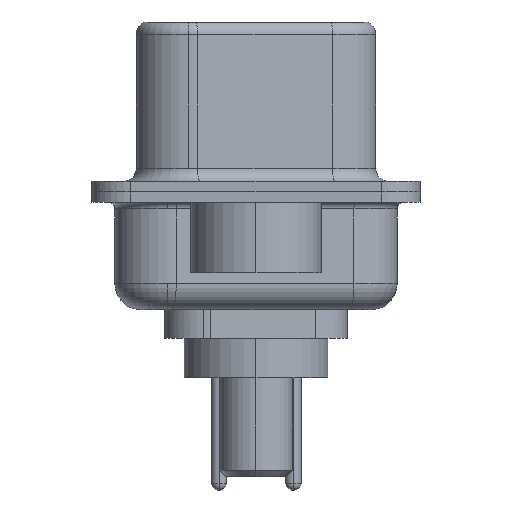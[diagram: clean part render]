
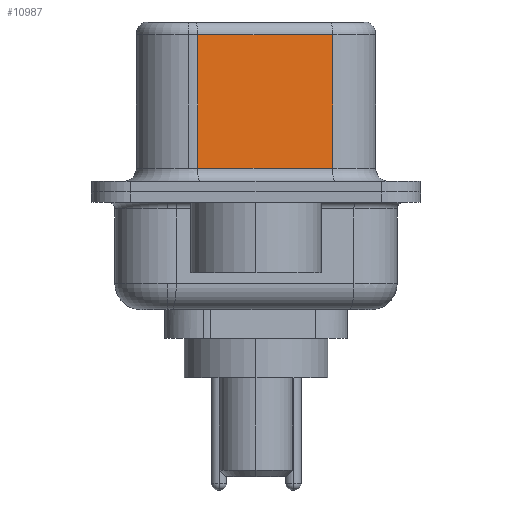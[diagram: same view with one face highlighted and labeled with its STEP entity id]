
A CAD part, left-side view. The second image highlights one B-rep face of the part: STEP entity #10987.
In plain terms, the highlighted planar face has unit normal (-0.985, -0.174, 0).
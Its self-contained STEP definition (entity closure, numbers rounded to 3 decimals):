
#9 = DIRECTION ( 'NONE',  ( -0.174, 0.985, 0. ) ) ;
#529 = FACE_OUTER_BOUND ( 'NONE', #4240, .T. ) ;
#559 = EDGE_CURVE ( 'NONE', #6951, #2837, #6944, .T. ) ;
#619 = VECTOR ( 'NONE', #14401, 1000. ) ;
#882 = DIRECTION ( 'NONE',  ( 0., 0., -1. ) ) ;
#1055 = LINE ( 'NONE', #1726, #619 ) ;
#1592 = EDGE_CURVE ( 'NONE', #12579, #16629, #1055, .T. ) ;
#1726 = CARTESIAN_POINT ( 'NONE',  ( 4.565, -2.927, 6.02 ) ) ;
#2046 = EDGE_CURVE ( 'NONE', #16629, #6951, #2813, .T. ) ;
#2109 = VECTOR ( 'NONE', #8975, 1000. ) ;
#2813 = LINE ( 'NONE', #11644, #14610 ) ;
#2837 = VERTEX_POINT ( 'NONE', #13193 ) ;
#2959 = CARTESIAN_POINT ( 'NONE',  ( 4.565, -2.927, 6.02 ) ) ;
#4240 = EDGE_LOOP ( 'NONE', ( #15422, #6058, #6425, #6544 ) ) ;
#4290 = DIRECTION ( 'NONE',  ( 0.174, -0.985, 0. ) ) ;
#5645 = PLANE ( 'NONE',  #6758 ) ;
#6058 = ORIENTED_EDGE ( 'NONE', *, *, #1592, .T. ) ;
#6401 = LINE ( 'NONE', #15905, #2109 ) ;
#6425 = ORIENTED_EDGE ( 'NONE', *, *, #2046, .T. ) ;
#6544 = ORIENTED_EDGE ( 'NONE', *, *, #559, .T. ) ;
#6758 = AXIS2_PLACEMENT_3D ( 'NONE', #7175, #8669, #9 ) ;
#6944 = LINE ( 'NONE', #12833, #16859 ) ;
#6951 = VERTEX_POINT ( 'NONE', #14210 ) ;
#7175 = CARTESIAN_POINT ( 'NONE',  ( 4.565, -2.927, 6.52 ) ) ;
#8323 = EDGE_CURVE ( 'NONE', #12579, #2837, #6401, .T. ) ;
#8669 = DIRECTION ( 'NONE',  ( 0.985, 0.174, 0. ) ) ;
#8975 = DIRECTION ( 'NONE',  ( 0., 0., -1. ) ) ;
#10987 = ADVANCED_FACE ( 'NONE', ( #529 ), #5645, .F. ) ;
#11644 = CARTESIAN_POINT ( 'NONE',  ( 3.655, 2.233, 6.52 ) ) ;
#12579 = VERTEX_POINT ( 'NONE', #2959 ) ;
#12833 = CARTESIAN_POINT ( 'NONE',  ( 4.565, -2.927, 0.9 ) ) ;
#13193 = CARTESIAN_POINT ( 'NONE',  ( 4.565, -2.927, 0.9 ) ) ;
#14210 = CARTESIAN_POINT ( 'NONE',  ( 3.655, 2.233, 0.9 ) ) ;
#14401 = DIRECTION ( 'NONE',  ( -0.174, 0.985, 0. ) ) ;
#14610 = VECTOR ( 'NONE', #882, 1000. ) ;
#15422 = ORIENTED_EDGE ( 'NONE', *, *, #8323, .F. ) ;
#15905 = CARTESIAN_POINT ( 'NONE',  ( 4.565, -2.927, 6.52 ) ) ;
#16629 = VERTEX_POINT ( 'NONE', #17345 ) ;
#16859 = VECTOR ( 'NONE', #4290, 1000. ) ;
#17345 = CARTESIAN_POINT ( 'NONE',  ( 3.655, 2.233, 6.02 ) ) ;
